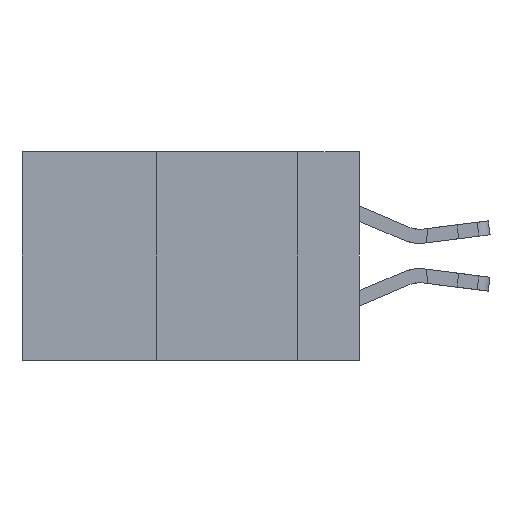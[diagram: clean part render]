
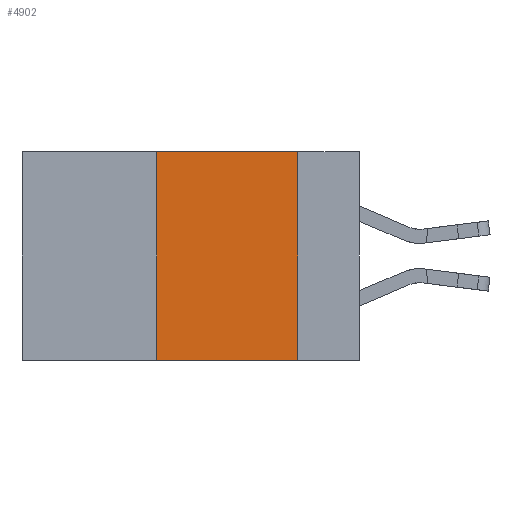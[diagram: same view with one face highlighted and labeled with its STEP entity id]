
A CAD part, left-side view. The second image highlights one B-rep face of the part: STEP entity #4902.
In plain terms, the highlighted planar face has unit normal (-1, 0, 0).
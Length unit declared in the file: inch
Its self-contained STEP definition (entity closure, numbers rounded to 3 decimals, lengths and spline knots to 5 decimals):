
#1148 = VECTOR ( 'NONE', #3709, 39.37008 ) ;
#1159 = DIRECTION ( 'NONE',  ( 0., 0., -1. ) ) ;
#2039 = CARTESIAN_POINT ( 'NONE',  ( 0., 0.6, 0. ) ) ;
#2337 = VERTEX_POINT ( 'NONE', #2894 ) ;
#2894 = CARTESIAN_POINT ( 'NONE',  ( 0., 0.36, 0. ) ) ;
#3133 = CARTESIAN_POINT ( 'NONE',  ( 0., 0.36, -0.37 ) ) ;
#3689 = DIRECTION ( 'NONE',  ( 1., 0., 0. ) ) ;
#3709 = DIRECTION ( 'NONE',  ( 0., -1., 0. ) ) ;
#4902 = ADVANCED_FACE ( 'NONE', ( #8386 ), #17054, .F. ) ;
#5019 = EDGE_CURVE ( 'NONE', #8307, #6469, #7758, .T. ) ;
#5257 = CARTESIAN_POINT ( 'NONE',  ( 0., 0.6, 0. ) ) ;
#5785 = DIRECTION ( 'NONE',  ( 0., 0., 1. ) ) ;
#5870 = ORIENTED_EDGE ( 'NONE', *, *, #11999, .F. ) ;
#6469 = VERTEX_POINT ( 'NONE', #10582 ) ;
#7758 = LINE ( 'NONE', #12794, #1148 ) ;
#8307 = VERTEX_POINT ( 'NONE', #3133 ) ;
#8386 = FACE_OUTER_BOUND ( 'NONE', #13952, .T. ) ;
#9432 = LINE ( 'NONE', #12685, #16327 ) ;
#9779 = CARTESIAN_POINT ( 'NONE',  ( 0., 0.36, 0. ) ) ;
#10582 = CARTESIAN_POINT ( 'NONE',  ( 0., 0.11, -0.37 ) ) ;
#11397 = AXIS2_PLACEMENT_3D ( 'NONE', #5257, #3689, #1159 ) ;
#11999 = EDGE_CURVE ( 'NONE', #16894, #6469, #9432, .T. ) ;
#12685 = CARTESIAN_POINT ( 'NONE',  ( 0., 0.11, 0. ) ) ;
#12758 = VECTOR ( 'NONE', #5785, 39.37008 ) ;
#12769 = LINE ( 'NONE', #2039, #14688 ) ;
#12794 = CARTESIAN_POINT ( 'NONE',  ( 0., 0.6, -0.37 ) ) ;
#13199 = CARTESIAN_POINT ( 'NONE',  ( 0., 0.11, 0. ) ) ;
#13575 = ORIENTED_EDGE ( 'NONE', *, *, #5019, .T. ) ;
#13952 = EDGE_LOOP ( 'NONE', ( #5870, #15790, #16877, #13575 ) ) ;
#14688 = VECTOR ( 'NONE', #15468, 39.37008 ) ;
#14952 = EDGE_CURVE ( 'NONE', #2337, #16894, #12769, .T. ) ;
#15468 = DIRECTION ( 'NONE',  ( 0., -1., 0. ) ) ;
#15474 = DIRECTION ( 'NONE',  ( 0., 0., -1. ) ) ;
#15790 = ORIENTED_EDGE ( 'NONE', *, *, #14952, .F. ) ;
#16174 = EDGE_CURVE ( 'NONE', #8307, #2337, #16747, .T. ) ;
#16327 = VECTOR ( 'NONE', #15474, 39.37008 ) ;
#16747 = LINE ( 'NONE', #9779, #12758 ) ;
#16877 = ORIENTED_EDGE ( 'NONE', *, *, #16174, .F. ) ;
#16894 = VERTEX_POINT ( 'NONE', #13199 ) ;
#17054 = PLANE ( 'NONE',  #11397 ) ;
